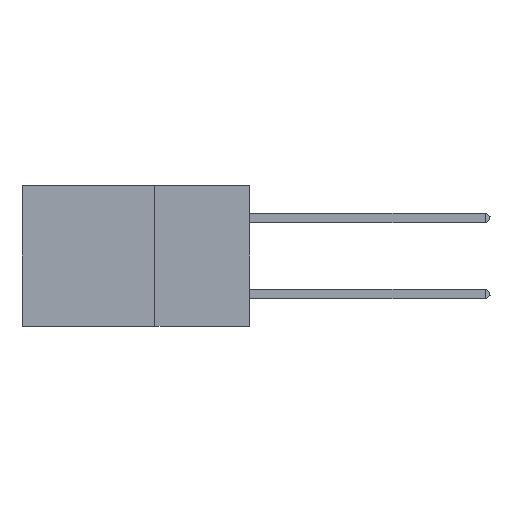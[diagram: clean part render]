
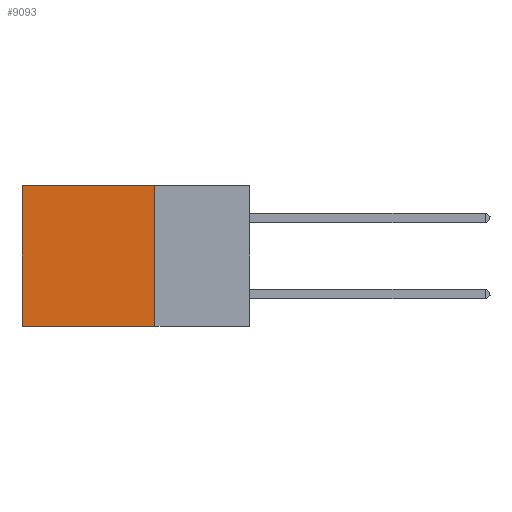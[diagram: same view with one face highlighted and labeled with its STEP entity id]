
A CAD part, left-side view. The second image highlights one B-rep face of the part: STEP entity #9093.
In plain terms, the highlighted planar face has unit normal (-1, 0, 0).
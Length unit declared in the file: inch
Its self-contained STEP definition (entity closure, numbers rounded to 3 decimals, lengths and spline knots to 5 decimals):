
#95 = VERTEX_POINT ( 'NONE', #27734 ) ;
#1209 = ORIENTED_EDGE ( 'NONE', *, *, #6513, .F. ) ;
#1998 = CARTESIAN_POINT ( 'NONE',  ( 0.2875, 0.6, 0. ) ) ;
#4112 = DIRECTION ( 'NONE',  ( 0., 0., -1. ) ) ;
#5002 = CARTESIAN_POINT ( 'NONE',  ( 0.2875, 0.25, -0.37 ) ) ;
#5905 = AXIS2_PLACEMENT_3D ( 'NONE', #16801, #28267, #10111 ) ;
#6513 = EDGE_CURVE ( 'NONE', #19066, #95, #27917, .T. ) ;
#6764 = ORIENTED_EDGE ( 'NONE', *, *, #11138, .T. ) ;
#7425 = DIRECTION ( 'NONE',  ( 0., 1., 0. ) ) ;
#7710 = ORIENTED_EDGE ( 'NONE', *, *, #21021, .T. ) ;
#9093 = ADVANCED_FACE ( 'NONE', ( #18469 ), #28168, .F. ) ;
#9769 = VECTOR ( 'NONE', #4112, 39.37008 ) ;
#10111 = DIRECTION ( 'NONE',  ( 0., 0., -1. ) ) ;
#10141 = LINE ( 'NONE', #18815, #12613 ) ;
#11138 = EDGE_CURVE ( 'NONE', #20827, #95, #23030, .T. ) ;
#11722 = CARTESIAN_POINT ( 'NONE',  ( 0.2875, 0.25, 0. ) ) ;
#12314 = CARTESIAN_POINT ( 'NONE',  ( 0.2875, 0.25, 0. ) ) ;
#12613 = VECTOR ( 'NONE', #7425, 39.37008 ) ;
#13699 = LINE ( 'NONE', #12314, #22698 ) ;
#14269 = CARTESIAN_POINT ( 'NONE',  ( 0.2875, 0.25, -0.37 ) ) ;
#16801 = CARTESIAN_POINT ( 'NONE',  ( 0.2875, 0.25, 0. ) ) ;
#16932 = DIRECTION ( 'NONE',  ( 0., 0., -1. ) ) ;
#17482 = VECTOR ( 'NONE', #23416, 39.37008 ) ;
#18469 = FACE_OUTER_BOUND ( 'NONE', #26666, .T. ) ;
#18815 = CARTESIAN_POINT ( 'NONE',  ( 0.2875, 0.25, 0. ) ) ;
#19066 = VERTEX_POINT ( 'NONE', #5002 ) ;
#19995 = ORIENTED_EDGE ( 'NONE', *, *, #27075, .F. ) ;
#20827 = VERTEX_POINT ( 'NONE', #24961 ) ;
#21021 = EDGE_CURVE ( 'NONE', #23487, #20827, #10141, .T. ) ;
#22698 = VECTOR ( 'NONE', #16932, 39.37008 ) ;
#23030 = LINE ( 'NONE', #1998, #9769 ) ;
#23416 = DIRECTION ( 'NONE',  ( 0., 1., 0. ) ) ;
#23487 = VERTEX_POINT ( 'NONE', #11722 ) ;
#24961 = CARTESIAN_POINT ( 'NONE',  ( 0.2875, 0.6, 0. ) ) ;
#26666 = EDGE_LOOP ( 'NONE', ( #6764, #1209, #19995, #7710 ) ) ;
#27075 = EDGE_CURVE ( 'NONE', #23487, #19066, #13699, .T. ) ;
#27734 = CARTESIAN_POINT ( 'NONE',  ( 0.2875, 0.6, -0.37 ) ) ;
#27917 = LINE ( 'NONE', #14269, #17482 ) ;
#28168 = PLANE ( 'NONE',  #5905 ) ;
#28267 = DIRECTION ( 'NONE',  ( 1., 0., 0. ) ) ;
